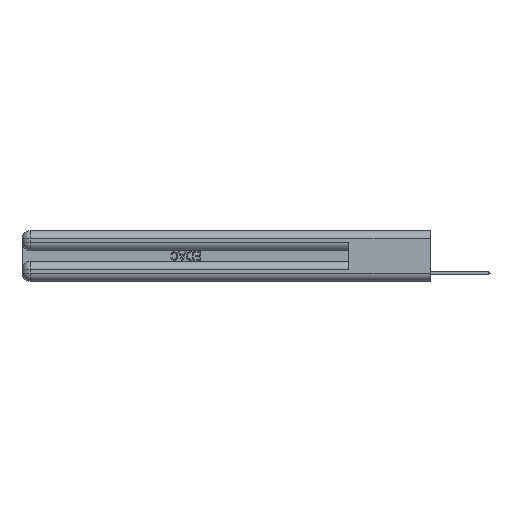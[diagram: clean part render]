
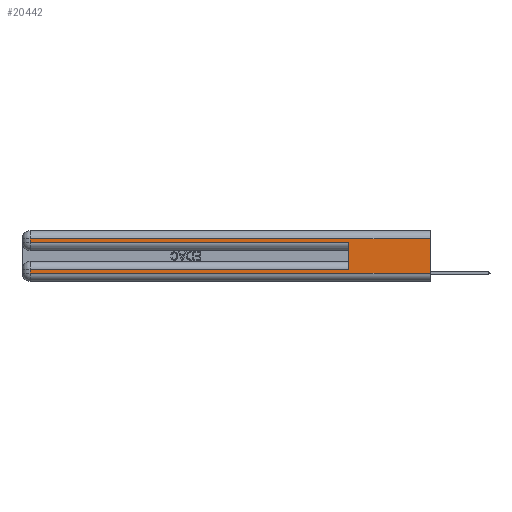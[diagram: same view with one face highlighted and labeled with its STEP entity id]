
A CAD part, left-side view. The second image highlights one B-rep face of the part: STEP entity #20442.
In plain terms, the highlighted planar face has unit normal (-1, 0, 0).
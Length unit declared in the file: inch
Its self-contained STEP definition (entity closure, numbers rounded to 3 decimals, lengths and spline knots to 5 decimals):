
#95 = VECTOR ( 'NONE', #21582, 39.37008 ) ;
#460 = CARTESIAN_POINT ( 'NONE',  ( 0., 0., 0.285 ) ) ;
#875 = EDGE_CURVE ( 'NONE', #13742, #22046, #26754, .T. ) ;
#954 = CARTESIAN_POINT ( 'NONE',  ( 0., 2.94, 0.285 ) ) ;
#1084 = DIRECTION ( 'NONE',  ( 0., -1., 0. ) ) ;
#1341 = LINE ( 'NONE', #5864, #10008 ) ;
#2026 = DIRECTION ( 'NONE',  ( 0., 1., 0. ) ) ;
#2081 = VERTEX_POINT ( 'NONE', #21872 ) ;
#3845 = VECTOR ( 'NONE', #4250, 39.37008 ) ;
#4250 = DIRECTION ( 'NONE',  ( 0., 0., 1. ) ) ;
#4602 = VECTOR ( 'NONE', #8415, 39.37008 ) ;
#5864 = CARTESIAN_POINT ( 'NONE',  ( 0., 2.94, 0.37 ) ) ;
#5886 = EDGE_CURVE ( 'NONE', #21173, #22046, #25396, .T. ) ;
#5917 = EDGE_CURVE ( 'NONE', #31212, #28171, #30737, .T. ) ;
#5923 = VECTOR ( 'NONE', #2026, 39.37008 ) ;
#6004 = CARTESIAN_POINT ( 'NONE',  ( 0., 0.6, 0.085 ) ) ;
#7303 = ORIENTED_EDGE ( 'NONE', *, *, #875, .F. ) ;
#7672 = VECTOR ( 'NONE', #15735, 39.37008 ) ;
#8415 = DIRECTION ( 'NONE',  ( 0., 0., -1. ) ) ;
#8954 = CARTESIAN_POINT ( 'NONE',  ( 0., 0., 0.06 ) ) ;
#9130 = EDGE_CURVE ( 'NONE', #15359, #28171, #31034, .T. ) ;
#9301 = FACE_OUTER_BOUND ( 'NONE', #27026, .T. ) ;
#9908 = VERTEX_POINT ( 'NONE', #26402 ) ;
#10008 = VECTOR ( 'NONE', #28547, 39.37008 ) ;
#10269 = VECTOR ( 'NONE', #1084, 39.37008 ) ;
#10861 = LINE ( 'NONE', #30759, #4602 ) ;
#11493 = CARTESIAN_POINT ( 'NONE',  ( 0., 2.94, 0.06 ) ) ;
#12517 = ORIENTED_EDGE ( 'NONE', *, *, #9130, .F. ) ;
#12648 = ORIENTED_EDGE ( 'NONE', *, *, #28907, .T. ) ;
#13742 = VERTEX_POINT ( 'NONE', #6004 ) ;
#14207 = CARTESIAN_POINT ( 'NONE',  ( 0., 0., 0.37 ) ) ;
#14446 = EDGE_CURVE ( 'NONE', #15359, #9908, #17570, .T. ) ;
#15359 = VERTEX_POINT ( 'NONE', #19397 ) ;
#15735 = DIRECTION ( 'NONE',  ( 0., -1., 0. ) ) ;
#15905 = CARTESIAN_POINT ( 'NONE',  ( 0., 0., 0.06 ) ) ;
#16173 = DIRECTION ( 'NONE',  ( 0., 0., -1. ) ) ;
#16482 = CARTESIAN_POINT ( 'NONE',  ( 0., 0.6, 0.145 ) ) ;
#17570 = LINE ( 'NONE', #20197, #17575 ) ;
#17575 = VECTOR ( 'NONE', #22650, 39.37008 ) ;
#18400 = EDGE_CURVE ( 'NONE', #2081, #31212, #1341, .T. ) ;
#19264 = DIRECTION ( 'NONE',  ( 1., 0., 0. ) ) ;
#19397 = CARTESIAN_POINT ( 'NONE',  ( 0., 0., 0.31 ) ) ;
#20197 = CARTESIAN_POINT ( 'NONE',  ( 0., 0., 0.31 ) ) ;
#20442 = ADVANCED_FACE ( 'NONE', ( #9301 ), #21393, .F. ) ;
#20555 = ORIENTED_EDGE ( 'NONE', *, *, #5917, .T. ) ;
#21173 = VERTEX_POINT ( 'NONE', #954 ) ;
#21268 = EDGE_CURVE ( 'NONE', #9908, #21173, #10861, .T. ) ;
#21337 = ORIENTED_EDGE ( 'NONE', *, *, #18400, .T. ) ;
#21393 = PLANE ( 'NONE',  #31656 ) ;
#21582 = DIRECTION ( 'NONE',  ( 0., 0., -1. ) ) ;
#21872 = CARTESIAN_POINT ( 'NONE',  ( 0., 2.94, 0.085 ) ) ;
#22046 = VERTEX_POINT ( 'NONE', #31616 ) ;
#22650 = DIRECTION ( 'NONE',  ( 0., 1., 0. ) ) ;
#22882 = ORIENTED_EDGE ( 'NONE', *, *, #21268, .T. ) ;
#25396 = LINE ( 'NONE', #460, #7672 ) ;
#26402 = CARTESIAN_POINT ( 'NONE',  ( 0., 2.94, 0.31 ) ) ;
#26484 = CARTESIAN_POINT ( 'NONE',  ( 0., 0., 0.37 ) ) ;
#26754 = LINE ( 'NONE', #16482, #3845 ) ;
#27026 = EDGE_LOOP ( 'NONE', ( #12517, #27277, #22882, #28783, #7303, #12648, #21337, #20555 ) ) ;
#27277 = ORIENTED_EDGE ( 'NONE', *, *, #14446, .T. ) ;
#28171 = VERTEX_POINT ( 'NONE', #8954 ) ;
#28547 = DIRECTION ( 'NONE',  ( 0., 0., -1. ) ) ;
#28783 = ORIENTED_EDGE ( 'NONE', *, *, #5886, .T. ) ;
#28907 = EDGE_CURVE ( 'NONE', #13742, #2081, #31514, .T. ) ;
#30737 = LINE ( 'NONE', #15905, #10269 ) ;
#30759 = CARTESIAN_POINT ( 'NONE',  ( 0., 2.94, 0.37 ) ) ;
#31034 = LINE ( 'NONE', #26484, #95 ) ;
#31212 = VERTEX_POINT ( 'NONE', #11493 ) ;
#31514 = LINE ( 'NONE', #32000, #5923 ) ;
#31616 = CARTESIAN_POINT ( 'NONE',  ( 0., 0.6, 0.285 ) ) ;
#31656 = AXIS2_PLACEMENT_3D ( 'NONE', #14207, #19264, #16173 ) ;
#32000 = CARTESIAN_POINT ( 'NONE',  ( 0., 0., 0.085 ) ) ;
